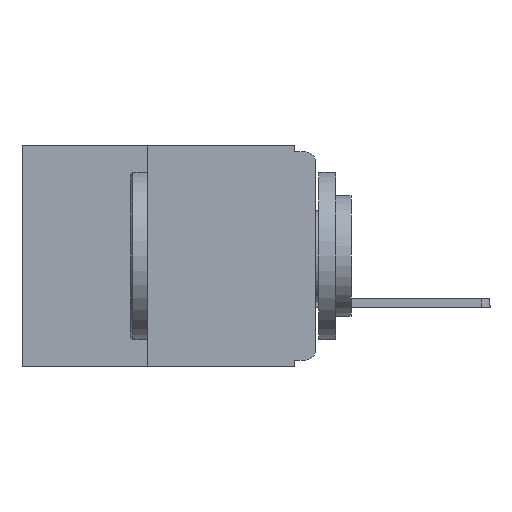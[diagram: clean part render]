
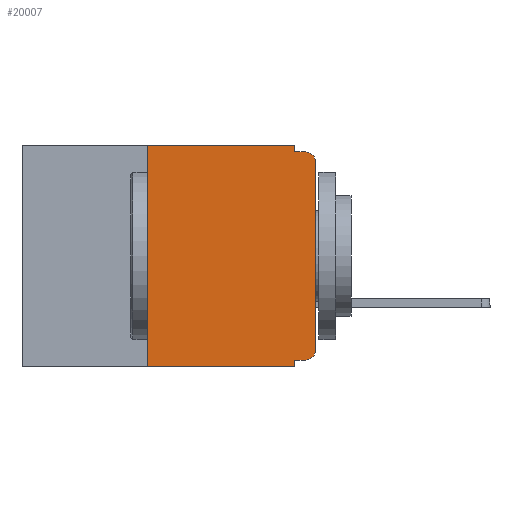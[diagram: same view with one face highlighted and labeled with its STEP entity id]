
A CAD part, left-side view. The second image highlights one B-rep face of the part: STEP entity #20007.
In plain terms, the highlighted planar face has unit normal (-1, 0, 0).
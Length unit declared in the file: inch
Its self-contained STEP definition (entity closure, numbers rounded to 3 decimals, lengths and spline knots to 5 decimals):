
#450 = CARTESIAN_POINT ( 'NONE',  ( 0., 0.015, -0.32 ) ) ;
#868 = VERTEX_POINT ( 'NONE', #450 ) ;
#880 = VECTOR ( 'NONE', #16540, 39.37008 ) ;
#881 = EDGE_CURVE ( 'NONE', #2782, #3368, #10502, .T. ) ;
#1251 = VECTOR ( 'NONE', #21588, 39.37008 ) ;
#2033 = CARTESIAN_POINT ( 'NONE',  ( 0., 0.437, 0. ) ) ;
#2563 = LINE ( 'NONE', #5805, #18369 ) ;
#2782 = VERTEX_POINT ( 'NONE', #10742 ) ;
#2959 = CARTESIAN_POINT ( 'NONE',  ( 0., 0., -0.305 ) ) ;
#3236 = CARTESIAN_POINT ( 'NONE',  ( 0., 0., -0.32 ) ) ;
#3368 = VERTEX_POINT ( 'NONE', #18203 ) ;
#3453 = EDGE_LOOP ( 'NONE', ( #10435, #22290, #7160, #5669, #25228, #18155, #5508, #20415, #10901, #8710 ) ) ;
#4606 = AXIS2_PLACEMENT_3D ( 'NONE', #9671, #23839, #11773 ) ;
#5353 = DIRECTION ( 'NONE',  ( 0., 1., 0. ) ) ;
#5432 = VERTEX_POINT ( 'NONE', #23217 ) ;
#5480 = VERTEX_POINT ( 'NONE', #2959 ) ;
#5508 = ORIENTED_EDGE ( 'NONE', *, *, #8244, .T. ) ;
#5590 = LINE ( 'NONE', #3236, #10473 ) ;
#5669 = ORIENTED_EDGE ( 'NONE', *, *, #15976, .F. ) ;
#5805 = CARTESIAN_POINT ( 'NONE',  ( 0., 0., 0. ) ) ;
#6496 = VERTEX_POINT ( 'NONE', #8339 ) ;
#6831 = CARTESIAN_POINT ( 'NONE',  ( 0., 0.015, -0.305 ) ) ;
#7160 = ORIENTED_EDGE ( 'NONE', *, *, #7970, .F. ) ;
#7300 = CARTESIAN_POINT ( 'NONE',  ( 0., 0.031, -0.01 ) ) ;
#7915 = DIRECTION ( 'NONE',  ( 0., 0., 1. ) ) ;
#7970 = EDGE_CURVE ( 'NONE', #12276, #6496, #11717, .T. ) ;
#8244 = EDGE_CURVE ( 'NONE', #12028, #3368, #26161, .T. ) ;
#8339 = CARTESIAN_POINT ( 'NONE',  ( 0., 0.015, -0.01 ) ) ;
#8710 = ORIENTED_EDGE ( 'NONE', *, *, #10118, .T. ) ;
#8945 = DIRECTION ( 'NONE',  ( 0., 0., -1. ) ) ;
#9074 = CIRCLE ( 'NONE', #15079, 0.015 ) ;
#9447 = LINE ( 'NONE', #13513, #1251 ) ;
#9495 = CARTESIAN_POINT ( 'NONE',  ( 0., 0.437, 0. ) ) ;
#9584 = PLANE ( 'NONE',  #13016 ) ;
#9671 = CARTESIAN_POINT ( 'NONE',  ( 0., 0.015, -0.025 ) ) ;
#10055 = VECTOR ( 'NONE', #10674, 39.37008 ) ;
#10118 = EDGE_CURVE ( 'NONE', #868, #5480, #9074, .T. ) ;
#10435 = ORIENTED_EDGE ( 'NONE', *, *, #15523, .T. ) ;
#10473 = VECTOR ( 'NONE', #5353, 39.37008 ) ;
#10502 = LINE ( 'NONE', #24405, #25998 ) ;
#10674 = DIRECTION ( 'NONE',  ( 0., -1., 0. ) ) ;
#10742 = CARTESIAN_POINT ( 'NONE',  ( 0., 0.031, -0.32 ) ) ;
#10901 = ORIENTED_EDGE ( 'NONE', *, *, #22375, .F. ) ;
#11688 = DIRECTION ( 'NONE',  ( 0., 0., -1. ) ) ;
#11717 = LINE ( 'NONE', #11886, #21145 ) ;
#11773 = DIRECTION ( 'NONE',  ( 0., 0., -1. ) ) ;
#11886 = CARTESIAN_POINT ( 'NONE',  ( 0., 0., -0.01 ) ) ;
#12028 = VERTEX_POINT ( 'NONE', #12692 ) ;
#12276 = VERTEX_POINT ( 'NONE', #7300 ) ;
#12692 = CARTESIAN_POINT ( 'NONE',  ( 0., 0.25, -0.33 ) ) ;
#12735 = EDGE_CURVE ( 'NONE', #12028, #22907, #19725, .T. ) ;
#12756 = CARTESIAN_POINT ( 'NONE',  ( 0., 0.437, -0.33 ) ) ;
#13016 = AXIS2_PLACEMENT_3D ( 'NONE', #9495, #23766, #11688 ) ;
#13513 = CARTESIAN_POINT ( 'NONE',  ( 0., 0.031, 0. ) ) ;
#15079 = AXIS2_PLACEMENT_3D ( 'NONE', #6831, #21095, #8945 ) ;
#15259 = CARTESIAN_POINT ( 'NONE',  ( 0., 0.25, -0.33 ) ) ;
#15523 = EDGE_CURVE ( 'NONE', #5480, #22306, #2563, .T. ) ;
#15976 = EDGE_CURVE ( 'NONE', #5432, #12276, #9447, .T. ) ;
#16540 = DIRECTION ( 'NONE',  ( 0., -1., 0. ) ) ;
#17382 = LINE ( 'NONE', #2033, #880 ) ;
#17555 = DIRECTION ( 'NONE',  ( 0., 0., -1. ) ) ;
#17710 = EDGE_CURVE ( 'NONE', #22306, #6496, #22075, .T. ) ;
#18155 = ORIENTED_EDGE ( 'NONE', *, *, #12735, .F. ) ;
#18203 = CARTESIAN_POINT ( 'NONE',  ( 0., 0.031, -0.33 ) ) ;
#18369 = VECTOR ( 'NONE', #7915, 39.37008 ) ;
#19072 = VECTOR ( 'NONE', #25323, 39.37008 ) ;
#19387 = FACE_OUTER_BOUND ( 'NONE', #3453, .T. ) ;
#19725 = LINE ( 'NONE', #15259, #19072 ) ;
#20007 = ADVANCED_FACE ( 'NONE', ( #19387 ), #9584, .F. ) ;
#20415 = ORIENTED_EDGE ( 'NONE', *, *, #881, .F. ) ;
#21095 = DIRECTION ( 'NONE',  ( -1., 0., 0. ) ) ;
#21145 = VECTOR ( 'NONE', #25969, 39.37008 ) ;
#21588 = DIRECTION ( 'NONE',  ( 0., 0., -1. ) ) ;
#21771 = CARTESIAN_POINT ( 'NONE',  ( 0., 0.25, 0. ) ) ;
#22075 = CIRCLE ( 'NONE', #4606, 0.015 ) ;
#22290 = ORIENTED_EDGE ( 'NONE', *, *, #17710, .T. ) ;
#22306 = VERTEX_POINT ( 'NONE', #25473 ) ;
#22375 = EDGE_CURVE ( 'NONE', #868, #2782, #5590, .T. ) ;
#22907 = VERTEX_POINT ( 'NONE', #21771 ) ;
#23217 = CARTESIAN_POINT ( 'NONE',  ( 0., 0.031, 0. ) ) ;
#23766 = DIRECTION ( 'NONE',  ( 1., 0., 0. ) ) ;
#23786 = EDGE_CURVE ( 'NONE', #22907, #5432, #17382, .T. ) ;
#23839 = DIRECTION ( 'NONE',  ( -1., 0., 0. ) ) ;
#24405 = CARTESIAN_POINT ( 'NONE',  ( 0., 0.031, -0.33 ) ) ;
#25228 = ORIENTED_EDGE ( 'NONE', *, *, #23786, .F. ) ;
#25323 = DIRECTION ( 'NONE',  ( 0., 0., 1. ) ) ;
#25473 = CARTESIAN_POINT ( 'NONE',  ( 0., 0., -0.025 ) ) ;
#25969 = DIRECTION ( 'NONE',  ( 0., -1., 0. ) ) ;
#25998 = VECTOR ( 'NONE', #17555, 39.37008 ) ;
#26161 = LINE ( 'NONE', #12756, #10055 ) ;
